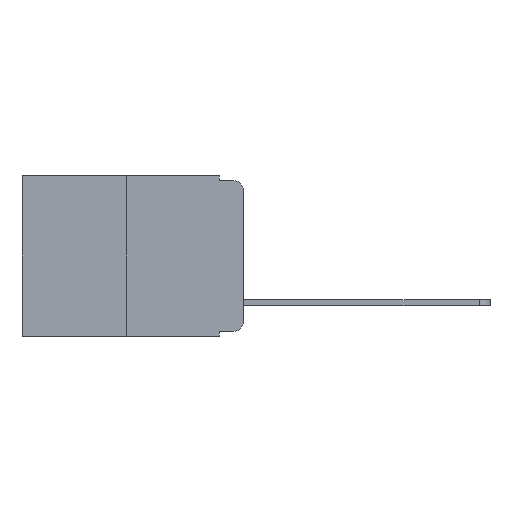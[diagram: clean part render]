
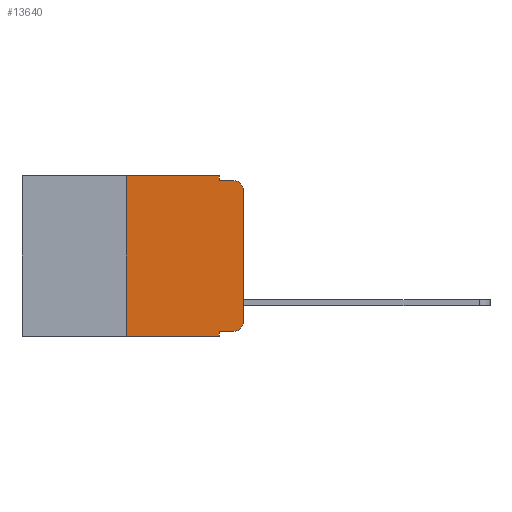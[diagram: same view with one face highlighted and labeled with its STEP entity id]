
A CAD part, left-side view. The second image highlights one B-rep face of the part: STEP entity #13640.
In plain terms, the highlighted planar face has unit normal (-1, 0, 0).
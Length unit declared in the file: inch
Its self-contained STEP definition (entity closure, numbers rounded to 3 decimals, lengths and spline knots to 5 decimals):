
#924 = DIRECTION ( 'NONE',  ( 0., 0., 1. ) ) ;
#1167 = CARTESIAN_POINT ( 'NONE',  ( 0., 0.25, 0. ) ) ;
#1213 = EDGE_CURVE ( 'NONE', #5656, #7058, #5043, .T. ) ;
#1628 = ORIENTED_EDGE ( 'NONE', *, *, #8231, .F. ) ;
#1671 = VECTOR ( 'NONE', #16256, 39.37008 ) ;
#1929 = EDGE_CURVE ( 'NONE', #8145, #17010, #9862, .T. ) ;
#2296 = EDGE_CURVE ( 'NONE', #4262, #18401, #11647, .T. ) ;
#2585 = ORIENTED_EDGE ( 'NONE', *, *, #1929, .T. ) ;
#3289 = EDGE_CURVE ( 'NONE', #6240, #4262, #8923, .T. ) ;
#3681 = DIRECTION ( 'NONE',  ( 1., 0., 0. ) ) ;
#3969 = VECTOR ( 'NONE', #5515, 39.37008 ) ;
#4044 = CARTESIAN_POINT ( 'NONE',  ( 0., 0.051, 0. ) ) ;
#4262 = VERTEX_POINT ( 'NONE', #14568 ) ;
#4444 = LINE ( 'NONE', #4044, #3969 ) ;
#4572 = VECTOR ( 'NONE', #6163, 39.37008 ) ;
#4989 = VECTOR ( 'NONE', #14012, 39.37008 ) ;
#5043 = LINE ( 'NONE', #15139, #4572 ) ;
#5255 = EDGE_CURVE ( 'NONE', #6240, #17010, #4444, .T. ) ;
#5515 = DIRECTION ( 'NONE',  ( 0., 0., -1. ) ) ;
#5561 = ORIENTED_EDGE ( 'NONE', *, *, #7252, .F. ) ;
#5656 = VERTEX_POINT ( 'NONE', #1167 ) ;
#6040 = ORIENTED_EDGE ( 'NONE', *, *, #6248, .F. ) ;
#6163 = DIRECTION ( 'NONE',  ( 0., -1., 0. ) ) ;
#6240 = VERTEX_POINT ( 'NONE', #11266 ) ;
#6248 = EDGE_CURVE ( 'NONE', #8145, #5656, #15079, .T. ) ;
#6969 = ORIENTED_EDGE ( 'NONE', *, *, #3289, .T. ) ;
#6984 = DIRECTION ( 'NONE',  ( 0., -1., 0. ) ) ;
#7058 = VERTEX_POINT ( 'NONE', #17137 ) ;
#7252 = EDGE_CURVE ( 'NONE', #7058, #18166, #9916, .T. ) ;
#7704 = CARTESIAN_POINT ( 'NONE',  ( 0., 0.02, -0.03 ) ) ;
#7893 = VECTOR ( 'NONE', #924, 39.37008 ) ;
#8145 = VERTEX_POINT ( 'NONE', #9699 ) ;
#8231 = EDGE_CURVE ( 'NONE', #18166, #12228, #17635, .T. ) ;
#8416 = CARTESIAN_POINT ( 'NONE',  ( 0., 0.25, 0. ) ) ;
#8905 = AXIS2_PLACEMENT_3D ( 'NONE', #7704, #17650, #9189 ) ;
#8923 = LINE ( 'NONE', #12918, #4989 ) ;
#9189 = DIRECTION ( 'NONE',  ( 0., 0., -1. ) ) ;
#9680 = VECTOR ( 'NONE', #6984, 39.37008 ) ;
#9699 = CARTESIAN_POINT ( 'NONE',  ( 0., 0.25, -0.343 ) ) ;
#9794 = DIRECTION ( 'NONE',  ( 0., -1., 0. ) ) ;
#9862 = LINE ( 'NONE', #10047, #16931 ) ;
#9916 = LINE ( 'NONE', #13291, #16979 ) ;
#10047 = CARTESIAN_POINT ( 'NONE',  ( 0., 0.473, -0.343 ) ) ;
#10522 = EDGE_LOOP ( 'NONE', ( #12427, #16591, #1628, #5561, #13319, #6040, #2585, #14213, #6969, #10873 ) ) ;
#10873 = ORIENTED_EDGE ( 'NONE', *, *, #2296, .T. ) ;
#10878 = CARTESIAN_POINT ( 'NONE',  ( 0., 0.051, -0.343 ) ) ;
#11157 = EDGE_CURVE ( 'NONE', #13043, #12228, #14287, .T. ) ;
#11266 = CARTESIAN_POINT ( 'NONE',  ( 0., 0.051, -0.333 ) ) ;
#11605 = CARTESIAN_POINT ( 'NONE',  ( 0., 0., -0.313 ) ) ;
#11647 = CIRCLE ( 'NONE', #12621, 0.02 ) ;
#11930 = DIRECTION ( 'NONE',  ( 0., 0., -1. ) ) ;
#12123 = EDGE_CURVE ( 'NONE', #18401, #13043, #17068, .T. ) ;
#12228 = VERTEX_POINT ( 'NONE', #13694 ) ;
#12427 = ORIENTED_EDGE ( 'NONE', *, *, #12123, .T. ) ;
#12453 = PLANE ( 'NONE',  #14700 ) ;
#12621 = AXIS2_PLACEMENT_3D ( 'NONE', #17263, #17258, #17238 ) ;
#12918 = CARTESIAN_POINT ( 'NONE',  ( 0., 0.051, -0.333 ) ) ;
#13043 = VERTEX_POINT ( 'NONE', #16876 ) ;
#13291 = CARTESIAN_POINT ( 'NONE',  ( 0., 0.051, 0. ) ) ;
#13319 = ORIENTED_EDGE ( 'NONE', *, *, #1213, .F. ) ;
#13640 = ADVANCED_FACE ( 'NONE', ( #15287 ), #12453, .F. ) ;
#13694 = CARTESIAN_POINT ( 'NONE',  ( 0., 0.02, -0.01 ) ) ;
#13892 = DIRECTION ( 'NONE',  ( 0., 0., -1. ) ) ;
#14012 = DIRECTION ( 'NONE',  ( 0., -1., 0. ) ) ;
#14201 = CARTESIAN_POINT ( 'NONE',  ( 0., 0.051, -0.01 ) ) ;
#14213 = ORIENTED_EDGE ( 'NONE', *, *, #5255, .F. ) ;
#14287 = CIRCLE ( 'NONE', #8905, 0.02 ) ;
#14568 = CARTESIAN_POINT ( 'NONE',  ( 0., 0.02, -0.333 ) ) ;
#14700 = AXIS2_PLACEMENT_3D ( 'NONE', #16621, #3681, #13892 ) ;
#14872 = CARTESIAN_POINT ( 'NONE',  ( 0., 0., 0. ) ) ;
#15079 = LINE ( 'NONE', #8416, #7893 ) ;
#15139 = CARTESIAN_POINT ( 'NONE',  ( 0., 0.473, 0. ) ) ;
#15204 = CARTESIAN_POINT ( 'NONE',  ( 0., 0.051, -0.01 ) ) ;
#15287 = FACE_OUTER_BOUND ( 'NONE', #10522, .T. ) ;
#16256 = DIRECTION ( 'NONE',  ( 0., 0., 1. ) ) ;
#16591 = ORIENTED_EDGE ( 'NONE', *, *, #11157, .T. ) ;
#16621 = CARTESIAN_POINT ( 'NONE',  ( 0., 0.473, 0. ) ) ;
#16876 = CARTESIAN_POINT ( 'NONE',  ( 0., 0., -0.03 ) ) ;
#16931 = VECTOR ( 'NONE', #9794, 39.37008 ) ;
#16979 = VECTOR ( 'NONE', #11930, 39.37008 ) ;
#17010 = VERTEX_POINT ( 'NONE', #10878 ) ;
#17068 = LINE ( 'NONE', #14872, #1671 ) ;
#17137 = CARTESIAN_POINT ( 'NONE',  ( 0., 0.051, 0. ) ) ;
#17238 = DIRECTION ( 'NONE',  ( 0., 0., -1. ) ) ;
#17258 = DIRECTION ( 'NONE',  ( -1., 0., 0. ) ) ;
#17263 = CARTESIAN_POINT ( 'NONE',  ( 0., 0.02, -0.313 ) ) ;
#17635 = LINE ( 'NONE', #14201, #9680 ) ;
#17650 = DIRECTION ( 'NONE',  ( -1., 0., 0. ) ) ;
#18166 = VERTEX_POINT ( 'NONE', #15204 ) ;
#18401 = VERTEX_POINT ( 'NONE', #11605 ) ;
